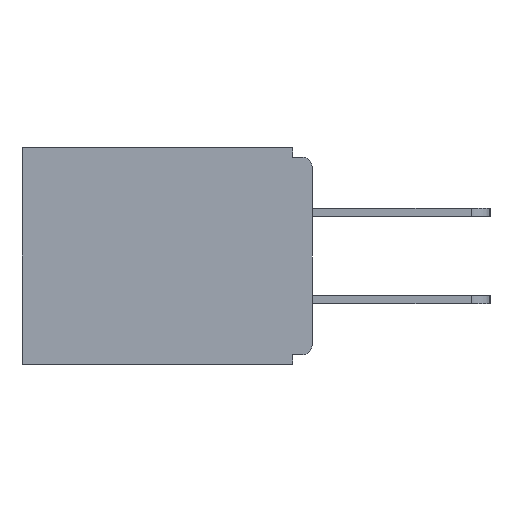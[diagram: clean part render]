
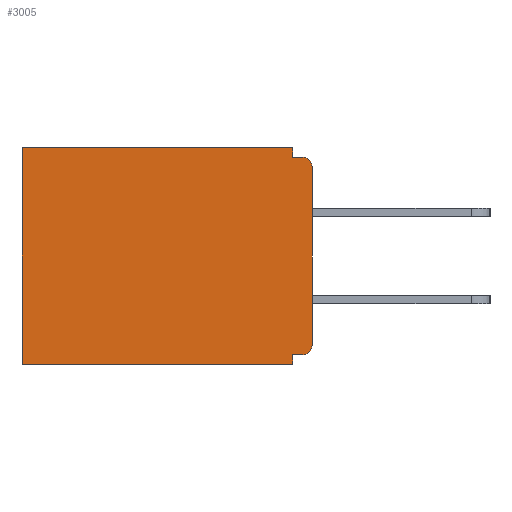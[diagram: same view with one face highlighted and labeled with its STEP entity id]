
A CAD part, left-side view. The second image highlights one B-rep face of the part: STEP entity #3005.
In plain terms, the highlighted planar face has unit normal (-1, 0, 0).
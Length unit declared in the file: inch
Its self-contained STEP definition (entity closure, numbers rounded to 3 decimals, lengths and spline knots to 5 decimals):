
#166 = CIRCLE ( 'NONE', #17451, 0.015 ) ;
#677 = EDGE_CURVE ( 'NONE', #20447, #15020, #7104, .T. ) ;
#843 = ORIENTED_EDGE ( 'NONE', *, *, #677, .F. ) ;
#952 = CARTESIAN_POINT ( 'NONE',  ( 0.298, 0.015, -0.313 ) ) ;
#1022 = DIRECTION ( 'NONE',  ( 0., 0., -1. ) ) ;
#1115 = CARTESIAN_POINT ( 'NONE',  ( 0.298, 0.46, 0. ) ) ;
#1585 = CARTESIAN_POINT ( 'NONE',  ( 0.298, 0., -0.015 ) ) ;
#1715 = VECTOR ( 'NONE', #15297, 39.37008 ) ;
#1734 = VECTOR ( 'NONE', #19127, 39.37008 ) ;
#1916 = AXIS2_PLACEMENT_3D ( 'NONE', #20579, #3518, #15482 ) ;
#2126 = VERTEX_POINT ( 'NONE', #5908 ) ;
#2639 = LINE ( 'NONE', #1585, #7168 ) ;
#2666 = ORIENTED_EDGE ( 'NONE', *, *, #21226, .F. ) ;
#3005 = ADVANCED_FACE ( 'NONE', ( #6197 ), #3580, .F. ) ;
#3148 = DIRECTION ( 'NONE',  ( 0., -1., 0. ) ) ;
#3518 = DIRECTION ( 'NONE',  ( 1., 0., 0. ) ) ;
#3580 = PLANE ( 'NONE',  #1916 ) ;
#4167 = EDGE_CURVE ( 'NONE', #5781, #8193, #16618, .T. ) ;
#5658 = DIRECTION ( 'NONE',  ( -1., 0., 0. ) ) ;
#5781 = VERTEX_POINT ( 'NONE', #20961 ) ;
#5908 = CARTESIAN_POINT ( 'NONE',  ( 0.298, 0.015, -0.015 ) ) ;
#6197 = FACE_OUTER_BOUND ( 'NONE', #12982, .T. ) ;
#6312 = CARTESIAN_POINT ( 'NONE',  ( 0.298, 0.031, -0.015 ) ) ;
#6487 = DIRECTION ( 'NONE',  ( 0., 0., -1. ) ) ;
#7104 = LINE ( 'NONE', #9925, #20280 ) ;
#7168 = VECTOR ( 'NONE', #3148, 39.37008 ) ;
#7350 = EDGE_CURVE ( 'NONE', #20447, #2126, #15510, .T. ) ;
#7495 = CARTESIAN_POINT ( 'NONE',  ( 0.298, 0.46, 0. ) ) ;
#7496 = AXIS2_PLACEMENT_3D ( 'NONE', #21655, #5658, #21577 ) ;
#7978 = VECTOR ( 'NONE', #18228, 39.37008 ) ;
#8193 = VERTEX_POINT ( 'NONE', #15363 ) ;
#8442 = ORIENTED_EDGE ( 'NONE', *, *, #10036, .F. ) ;
#8549 = VECTOR ( 'NONE', #14151, 39.37008 ) ;
#8613 = CARTESIAN_POINT ( 'NONE',  ( 0.298, 0., 0. ) ) ;
#8783 = VERTEX_POINT ( 'NONE', #11902 ) ;
#9414 = CARTESIAN_POINT ( 'NONE',  ( 0.298, 0.031, -0.343 ) ) ;
#9640 = EDGE_CURVE ( 'NONE', #13807, #15020, #166, .T. ) ;
#9925 = CARTESIAN_POINT ( 'NONE',  ( 0.298, 0., 0. ) ) ;
#10036 = EDGE_CURVE ( 'NONE', #8783, #15858, #14829, .T. ) ;
#10355 = ORIENTED_EDGE ( 'NONE', *, *, #18389, .F. ) ;
#10745 = CARTESIAN_POINT ( 'NONE',  ( 0.298, 0.031, -0.328 ) ) ;
#11120 = ORIENTED_EDGE ( 'NONE', *, *, #4167, .F. ) ;
#11457 = DIRECTION ( 'NONE',  ( 0., 0., -1. ) ) ;
#11523 = CARTESIAN_POINT ( 'NONE',  ( 0.298, 0.015, -0.328 ) ) ;
#11902 = CARTESIAN_POINT ( 'NONE',  ( 0.298, 0.031, 0. ) ) ;
#12982 = EDGE_LOOP ( 'NONE', ( #21810, #10355, #8442, #21751, #14060, #11120, #2666, #17919, #21005, #843 ) ) ;
#13057 = CARTESIAN_POINT ( 'NONE',  ( 0.298, 0., -0.313 ) ) ;
#13468 = LINE ( 'NONE', #8613, #1715 ) ;
#13663 = VECTOR ( 'NONE', #19530, 39.37008 ) ;
#13807 = VERTEX_POINT ( 'NONE', #11523 ) ;
#14060 = ORIENTED_EDGE ( 'NONE', *, *, #17823, .T. ) ;
#14151 = DIRECTION ( 'NONE',  ( 0., 1., 0. ) ) ;
#14829 = LINE ( 'NONE', #9414, #20192 ) ;
#15020 = VERTEX_POINT ( 'NONE', #13057 ) ;
#15297 = DIRECTION ( 'NONE',  ( 0., 1., 0. ) ) ;
#15363 = CARTESIAN_POINT ( 'NONE',  ( 0.298, 0.46, -0.343 ) ) ;
#15482 = DIRECTION ( 'NONE',  ( 0., 0., -1. ) ) ;
#15510 = CIRCLE ( 'NONE', #7496, 0.015 ) ;
#15858 = VERTEX_POINT ( 'NONE', #6312 ) ;
#16039 = CARTESIAN_POINT ( 'NONE',  ( 0.298, 0., -0.343 ) ) ;
#16066 = LINE ( 'NONE', #1115, #7978 ) ;
#16087 = LINE ( 'NONE', #19599, #13663 ) ;
#16290 = DIRECTION ( 'NONE',  ( -1., 0., 0. ) ) ;
#16452 = LINE ( 'NONE', #17180, #1734 ) ;
#16483 = CARTESIAN_POINT ( 'NONE',  ( 0.298, 0., -0.03 ) ) ;
#16618 = LINE ( 'NONE', #16039, #8549 ) ;
#17180 = CARTESIAN_POINT ( 'NONE',  ( 0.298, 0.031, -0.343 ) ) ;
#17451 = AXIS2_PLACEMENT_3D ( 'NONE', #952, #16290, #1022 ) ;
#17632 = EDGE_CURVE ( 'NONE', #13807, #18012, #16087, .T. ) ;
#17823 = EDGE_CURVE ( 'NONE', #18796, #8193, #16066, .T. ) ;
#17919 = ORIENTED_EDGE ( 'NONE', *, *, #17632, .F. ) ;
#18012 = VERTEX_POINT ( 'NONE', #10745 ) ;
#18228 = DIRECTION ( 'NONE',  ( 0., 0., -1. ) ) ;
#18389 = EDGE_CURVE ( 'NONE', #15858, #2126, #2639, .T. ) ;
#18796 = VERTEX_POINT ( 'NONE', #7495 ) ;
#19127 = DIRECTION ( 'NONE',  ( 0., 0., -1. ) ) ;
#19530 = DIRECTION ( 'NONE',  ( 0., 1., 0. ) ) ;
#19599 = CARTESIAN_POINT ( 'NONE',  ( 0.298, 0., -0.328 ) ) ;
#20192 = VECTOR ( 'NONE', #11457, 39.37008 ) ;
#20280 = VECTOR ( 'NONE', #6487, 39.37008 ) ;
#20447 = VERTEX_POINT ( 'NONE', #16483 ) ;
#20579 = CARTESIAN_POINT ( 'NONE',  ( 0.298, 0., 0. ) ) ;
#20961 = CARTESIAN_POINT ( 'NONE',  ( 0.298, 0.031, -0.343 ) ) ;
#21005 = ORIENTED_EDGE ( 'NONE', *, *, #9640, .T. ) ;
#21226 = EDGE_CURVE ( 'NONE', #18012, #5781, #16452, .T. ) ;
#21577 = DIRECTION ( 'NONE',  ( 0., 0., -1. ) ) ;
#21655 = CARTESIAN_POINT ( 'NONE',  ( 0.298, 0.015, -0.03 ) ) ;
#21751 = ORIENTED_EDGE ( 'NONE', *, *, #21826, .T. ) ;
#21810 = ORIENTED_EDGE ( 'NONE', *, *, #7350, .T. ) ;
#21826 = EDGE_CURVE ( 'NONE', #8783, #18796, #13468, .T. ) ;
